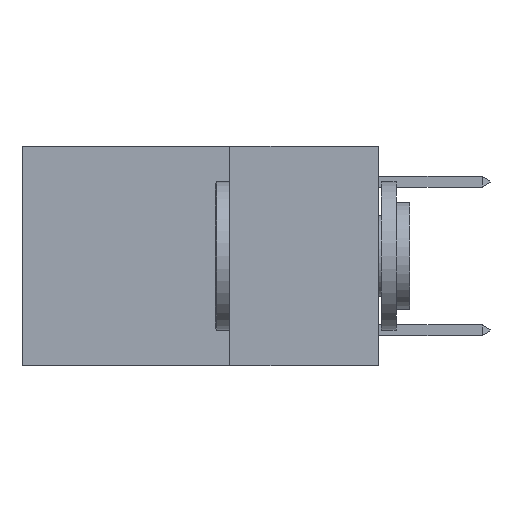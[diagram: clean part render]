
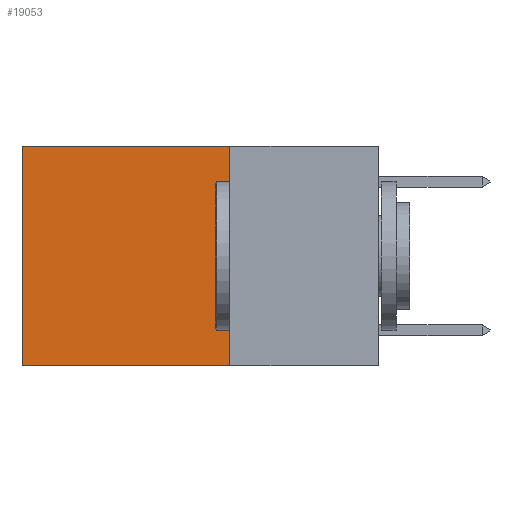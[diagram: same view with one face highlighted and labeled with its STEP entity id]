
A CAD part, left-side view. The second image highlights one B-rep face of the part: STEP entity #19053.
In plain terms, the highlighted planar face has unit normal (-1, 0, 0).
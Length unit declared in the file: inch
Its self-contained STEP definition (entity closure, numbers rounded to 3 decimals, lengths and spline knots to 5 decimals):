
#2005 = EDGE_LOOP ( 'NONE', ( #29138, #25992, #10047, #24436 ) ) ;
#2631 = EDGE_CURVE ( 'NONE', #15879, #3989, #29156, .T. ) ;
#3989 = VERTEX_POINT ( 'NONE', #16020 ) ;
#5010 = LINE ( 'NONE', #14329, #19477 ) ;
#5272 = VECTOR ( 'NONE', #20776, 39.37008 ) ;
#5752 = FACE_OUTER_BOUND ( 'NONE', #2005, .T. ) ;
#5910 = CARTESIAN_POINT ( 'NONE',  ( 0.2625, 0.25, 0. ) ) ;
#7415 = VERTEX_POINT ( 'NONE', #14081 ) ;
#9523 = DIRECTION ( 'NONE',  ( 0., 1., 0. ) ) ;
#9719 = DIRECTION ( 'NONE',  ( 0., 0., -1. ) ) ;
#10047 = ORIENTED_EDGE ( 'NONE', *, *, #20773, .F. ) ;
#10236 = VERTEX_POINT ( 'NONE', #26448 ) ;
#11252 = CARTESIAN_POINT ( 'NONE',  ( 0.2625, 0.6, 0. ) ) ;
#14081 = CARTESIAN_POINT ( 'NONE',  ( 0.2625, 0.25, 0. ) ) ;
#14329 = CARTESIAN_POINT ( 'NONE',  ( 0.2625, 0.25, 0. ) ) ;
#15264 = DIRECTION ( 'NONE',  ( 1., 0., 0. ) ) ;
#15879 = VERTEX_POINT ( 'NONE', #17149 ) ;
#16020 = CARTESIAN_POINT ( 'NONE',  ( 0.2625, 0.6, -0.37 ) ) ;
#17149 = CARTESIAN_POINT ( 'NONE',  ( 0.2625, 0.6, 0. ) ) ;
#17460 = VECTOR ( 'NONE', #9523, 39.37008 ) ;
#19053 = ADVANCED_FACE ( 'NONE', ( #5752 ), #26861, .F. ) ;
#19477 = VECTOR ( 'NONE', #9719, 39.37008 ) ;
#20108 = EDGE_CURVE ( 'NONE', #7415, #15879, #22769, .T. ) ;
#20773 = EDGE_CURVE ( 'NONE', #7415, #10236, #5010, .T. ) ;
#20776 = DIRECTION ( 'NONE',  ( 0., 1., 0. ) ) ;
#22769 = LINE ( 'NONE', #27515, #5272 ) ;
#23391 = EDGE_CURVE ( 'NONE', #10236, #3989, #23592, .T. ) ;
#23521 = VECTOR ( 'NONE', #27160, 39.37008 ) ;
#23592 = LINE ( 'NONE', #28473, #17460 ) ;
#24436 = ORIENTED_EDGE ( 'NONE', *, *, #20108, .T. ) ;
#24566 = DIRECTION ( 'NONE',  ( 0., 0., -1. ) ) ;
#25992 = ORIENTED_EDGE ( 'NONE', *, *, #23391, .F. ) ;
#26448 = CARTESIAN_POINT ( 'NONE',  ( 0.2625, 0.25, -0.37 ) ) ;
#26861 = PLANE ( 'NONE',  #29159 ) ;
#27160 = DIRECTION ( 'NONE',  ( 0., 0., -1. ) ) ;
#27515 = CARTESIAN_POINT ( 'NONE',  ( 0.2625, 0.25, 0. ) ) ;
#28473 = CARTESIAN_POINT ( 'NONE',  ( 0.2625, 0.25, -0.37 ) ) ;
#29138 = ORIENTED_EDGE ( 'NONE', *, *, #2631, .T. ) ;
#29156 = LINE ( 'NONE', #11252, #23521 ) ;
#29159 = AXIS2_PLACEMENT_3D ( 'NONE', #5910, #15264, #24566 ) ;
